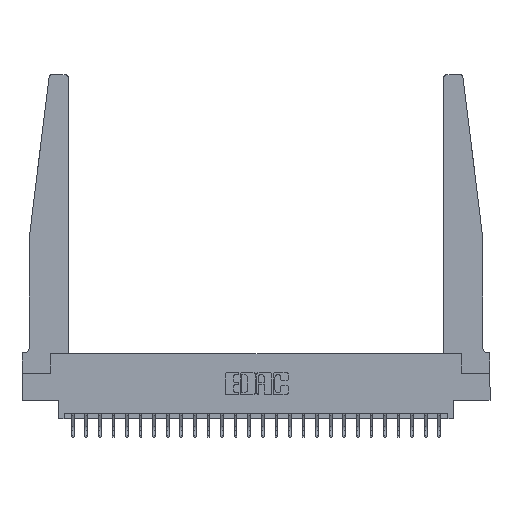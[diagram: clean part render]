
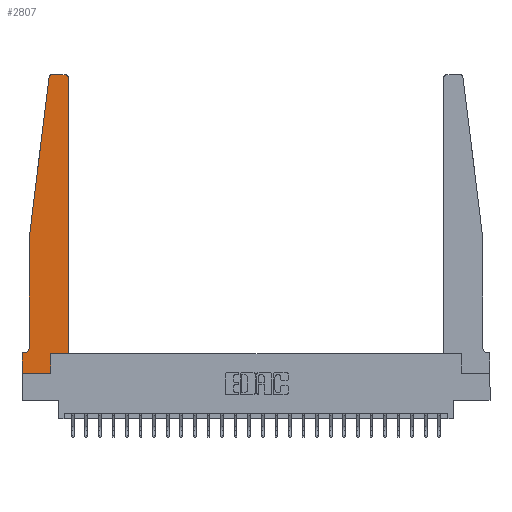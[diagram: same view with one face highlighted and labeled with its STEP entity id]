
A CAD part, top view. The second image highlights one B-rep face of the part: STEP entity #2807.
In plain terms, the highlighted planar face has unit normal (0, 0, 1).
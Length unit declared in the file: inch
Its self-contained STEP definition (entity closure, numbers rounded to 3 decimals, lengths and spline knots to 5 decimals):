
#450 = CARTESIAN_POINT ( 'NONE',  ( 0.395, 2.75, 0.37 ) ) ;
#1227 = CARTESIAN_POINT ( 'NONE',  ( 0.2605, 0., 0.37 ) ) ;
#1321 = CARTESIAN_POINT ( 'NONE',  ( 0., 0., 0.37 ) ) ;
#1387 = VECTOR ( 'NONE', #3783, 39.37008 ) ;
#1895 = CARTESIAN_POINT ( 'NONE',  ( 0., 0.1875, 0.37 ) ) ;
#1980 = DIRECTION ( 'NONE',  ( 1., 0., 0. ) ) ;
#2001 = LINE ( 'NONE', #23212, #1387 ) ;
#2069 = ORIENTED_EDGE ( 'NONE', *, *, #10526, .T. ) ;
#2266 = VERTEX_POINT ( 'NONE', #9931 ) ;
#2437 = CARTESIAN_POINT ( 'NONE',  ( 0.065, 1.25, 0.37 ) ) ;
#2477 = DIRECTION ( 'NONE',  ( -1., 0., 0. ) ) ;
#2807 = ADVANCED_FACE ( 'NONE', ( #15367 ), #9802, .T. ) ;
#3078 = EDGE_CURVE ( 'NONE', #4514, #16287, #9242, .T. ) ;
#3783 = DIRECTION ( 'NONE',  ( 0., 1., 0. ) ) ;
#4409 = CARTESIAN_POINT ( 'NONE',  ( 0.065, 0.1875, 0.37 ) ) ;
#4514 = VERTEX_POINT ( 'NONE', #12699 ) ;
#5129 = CARTESIAN_POINT ( 'NONE',  ( 0.24675, 2.72367, 0.37 ) ) ;
#5281 = VECTOR ( 'NONE', #18436, 39.37008 ) ;
#5630 = VERTEX_POINT ( 'NONE', #18263 ) ;
#5667 = CARTESIAN_POINT ( 'NONE',  ( 0.015, 0.1875, 0.37 ) ) ;
#6032 = LINE ( 'NONE', #25169, #15796 ) ;
#6287 = DIRECTION ( 'NONE',  ( 0., 0., 1. ) ) ;
#6618 = ORIENTED_EDGE ( 'NONE', *, *, #23784, .T. ) ;
#6757 = CARTESIAN_POINT ( 'NONE',  ( 0.425, 0.18, 0.37 ) ) ;
#6900 = CARTESIAN_POINT ( 'NONE',  ( 0.065, 1.25, 0.37 ) ) ;
#7486 = DIRECTION ( 'NONE',  ( -0.122, -0.992, 0. ) ) ;
#7567 = EDGE_CURVE ( 'NONE', #8221, #2266, #19426, .T. ) ;
#7769 = AXIS2_PLACEMENT_3D ( 'NONE', #1895, #13742, #1980 ) ;
#7913 = ORIENTED_EDGE ( 'NONE', *, *, #25117, .T. ) ;
#8221 = VERTEX_POINT ( 'NONE', #450 ) ;
#8259 = DIRECTION ( 'NONE',  ( -1., 0., 0. ) ) ;
#8455 = VECTOR ( 'NONE', #8259, 39.37008 ) ;
#8775 = CARTESIAN_POINT ( 'NONE',  ( 0.27653, 2.72, 0.37 ) ) ;
#9044 = ORIENTED_EDGE ( 'NONE', *, *, #23256, .T. ) ;
#9242 = LINE ( 'NONE', #6757, #5281 ) ;
#9433 = ORIENTED_EDGE ( 'NONE', *, *, #13184, .T. ) ;
#9449 = CARTESIAN_POINT ( 'NONE',  ( 0.015, 0.2375, 0.37 ) ) ;
#9793 = CARTESIAN_POINT ( 'NONE',  ( 0.2605, 0.18, 0.37 ) ) ;
#9802 = PLANE ( 'NONE',  #7769 ) ;
#9849 = ORIENTED_EDGE ( 'NONE', *, *, #3078, .T. ) ;
#9931 = CARTESIAN_POINT ( 'NONE',  ( 0.27653, 2.75, 0.37 ) ) ;
#10526 = EDGE_CURVE ( 'NONE', #14402, #4514, #21462, .T. ) ;
#10738 = DIRECTION ( 'NONE',  ( 1., 0., 0. ) ) ;
#10974 = AXIS2_PLACEMENT_3D ( 'NONE', #17970, #6287, #19908 ) ;
#11424 = DIRECTION ( 'NONE',  ( -1., 0., 0. ) ) ;
#11440 = CARTESIAN_POINT ( 'NONE',  ( 0.425, 0.18, 0.37 ) ) ;
#11743 = VECTOR ( 'NONE', #23072, 39.37008 ) ;
#12699 = CARTESIAN_POINT ( 'NONE',  ( 0.425, 0.18, 0.37 ) ) ;
#12878 = CIRCLE ( 'NONE', #16732, 0.05 ) ;
#13184 = EDGE_CURVE ( 'NONE', #21930, #19478, #12878, .T. ) ;
#13386 = CIRCLE ( 'NONE', #19551, 0.03 ) ;
#13742 = DIRECTION ( 'NONE',  ( 0., 0., 1. ) ) ;
#14185 = ORIENTED_EDGE ( 'NONE', *, *, #18714, .T. ) ;
#14402 = VERTEX_POINT ( 'NONE', #9793 ) ;
#14777 = CARTESIAN_POINT ( 'NONE',  ( 0.065, 0.2375, 0.37 ) ) ;
#14860 = ORIENTED_EDGE ( 'NONE', *, *, #17534, .T. ) ;
#15065 = DIRECTION ( 'NONE',  ( 0., -1., 0. ) ) ;
#15310 = CARTESIAN_POINT ( 'NONE',  ( 0.425, 2.72, 0.37 ) ) ;
#15367 = FACE_OUTER_BOUND ( 'NONE', #18050, .T. ) ;
#15476 = VECTOR ( 'NONE', #18126, 39.37008 ) ;
#15484 = VECTOR ( 'NONE', #2477, 39.37008 ) ;
#15516 = DIRECTION ( 'NONE',  ( 1., 0., 0. ) ) ;
#15680 = CARTESIAN_POINT ( 'NONE',  ( 0., 0., 0.37 ) ) ;
#15796 = VECTOR ( 'NONE', #15516, 39.37008 ) ;
#16287 = VERTEX_POINT ( 'NONE', #15310 ) ;
#16732 = AXIS2_PLACEMENT_3D ( 'NONE', #9449, #23060, #11424 ) ;
#16984 = ORIENTED_EDGE ( 'NONE', *, *, #7567, .T. ) ;
#17534 = EDGE_CURVE ( 'NONE', #5630, #24923, #18946, .T. ) ;
#17970 = CARTESIAN_POINT ( 'NONE',  ( 0.395, 2.72, 0.37 ) ) ;
#18050 = EDGE_LOOP ( 'NONE', ( #16984, #14185, #9044, #24946, #9433, #7913, #14860, #22929, #23476, #2069, #9849, #6618 ) ) ;
#18126 = DIRECTION ( 'NONE',  ( 0., -1., 0. ) ) ;
#18137 = VERTEX_POINT ( 'NONE', #5129 ) ;
#18263 = CARTESIAN_POINT ( 'NONE',  ( 0., 0.1875, 0.37 ) ) ;
#18337 = VECTOR ( 'NONE', #15065, 39.37008 ) ;
#18436 = DIRECTION ( 'NONE',  ( 0., 1., 0. ) ) ;
#18714 = EDGE_CURVE ( 'NONE', #2266, #18137, #13386, .T. ) ;
#18932 = LINE ( 'NONE', #19154, #24060 ) ;
#18946 = LINE ( 'NONE', #1321, #18337 ) ;
#19047 = EDGE_CURVE ( 'NONE', #19453, #14402, #2001, .T. ) ;
#19154 = CARTESIAN_POINT ( 'NONE',  ( 0.065, 1.25, 0.37 ) ) ;
#19426 = LINE ( 'NONE', #19920, #8455 ) ;
#19453 = VERTEX_POINT ( 'NONE', #1227 ) ;
#19478 = VERTEX_POINT ( 'NONE', #5667 ) ;
#19551 = AXIS2_PLACEMENT_3D ( 'NONE', #8775, #22386, #10738 ) ;
#19781 = EDGE_CURVE ( 'NONE', #23081, #21930, #21248, .T. ) ;
#19908 = DIRECTION ( 'NONE',  ( 1., 0., 0. ) ) ;
#19920 = CARTESIAN_POINT ( 'NONE',  ( 0.25, 2.75, 0.37 ) ) ;
#21248 = LINE ( 'NONE', #2437, #15476 ) ;
#21256 = LINE ( 'NONE', #4409, #15484 ) ;
#21462 = LINE ( 'NONE', #11440, #11743 ) ;
#21930 = VERTEX_POINT ( 'NONE', #14777 ) ;
#22386 = DIRECTION ( 'NONE',  ( 0., 0., 1. ) ) ;
#22929 = ORIENTED_EDGE ( 'NONE', *, *, #24880, .T. ) ;
#23060 = DIRECTION ( 'NONE',  ( 0., 0., -1. ) ) ;
#23072 = DIRECTION ( 'NONE',  ( 1., 0., 0. ) ) ;
#23081 = VERTEX_POINT ( 'NONE', #6900 ) ;
#23212 = CARTESIAN_POINT ( 'NONE',  ( 0.2605, 0.18, 0.37 ) ) ;
#23256 = EDGE_CURVE ( 'NONE', #18137, #23081, #18932, .T. ) ;
#23476 = ORIENTED_EDGE ( 'NONE', *, *, #19047, .T. ) ;
#23784 = EDGE_CURVE ( 'NONE', #16287, #8221, #24642, .T. ) ;
#24060 = VECTOR ( 'NONE', #7486, 39.37008 ) ;
#24642 = CIRCLE ( 'NONE', #10974, 0.03 ) ;
#24880 = EDGE_CURVE ( 'NONE', #24923, #19453, #6032, .T. ) ;
#24923 = VERTEX_POINT ( 'NONE', #15680 ) ;
#24946 = ORIENTED_EDGE ( 'NONE', *, *, #19781, .T. ) ;
#25117 = EDGE_CURVE ( 'NONE', #19478, #5630, #21256, .T. ) ;
#25169 = CARTESIAN_POINT ( 'NONE',  ( 0., 0., 0.37 ) ) ;
